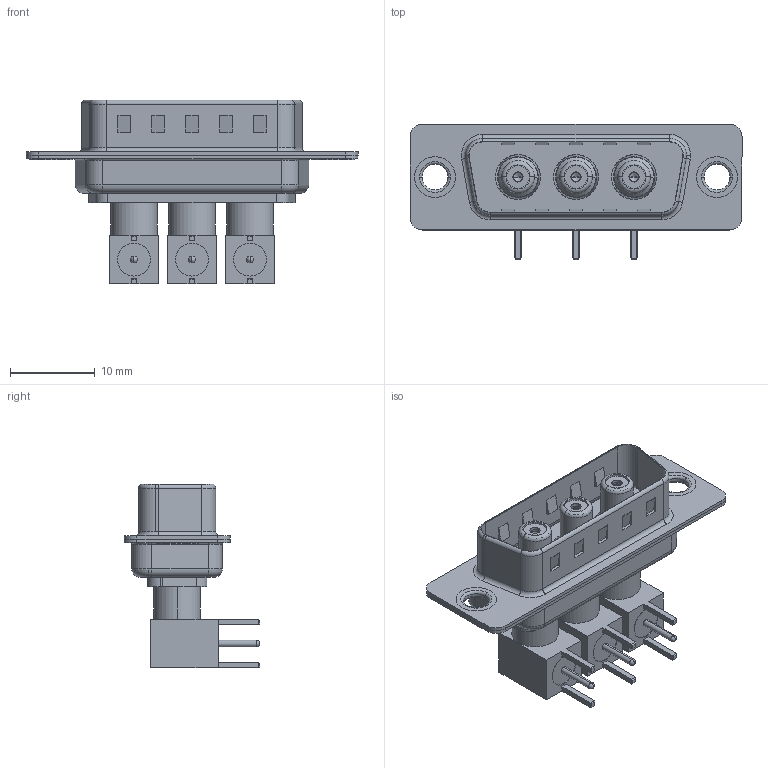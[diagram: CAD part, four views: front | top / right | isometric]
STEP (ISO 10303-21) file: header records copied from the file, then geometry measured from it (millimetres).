
FILE_DESCRIPTION (( 'STEP AP203' ), '1' );
FILE_NAME ('629-3W3-640-7T1.STEP', '2022-05-05T06:26:25', ( '' ), ( '' ), 'SwSTEP 2.0', 'SolidWorks 2020', '' );
FILE_SCHEMA (( 'CONFIG_CONTROL_DESIGN' ));
Length unit declared in the file: millimetre
Products named in the file (15): RA Back Shell; Locking Collar; Co-Ax Jack_RA PC Tail; 629-3W3-640-7T1; Co-Ax Jack Assy_RA; 629Combo Shell Rear_15 Contacts; Insulator RA Pin; Socket_RA; 629Combo Housing_3W3; 629Combo Thru Hole Rivet; Insulator Socket; Insulator Socket 2; 629Combo Shell Front_15 Contacts
Assembly tree (29 placements, depth 3):
  629-3W3-640-7T1
    629Combo Housing_3W3
    629Combo Shell Rear_15 Contacts
    629Combo Shell Front_15 Contacts
    629Combo Thru Hole Rivet  x2
    Co-Ax Jack Assy_RA
      Co-Ax Jack_RA PC Tail
      Insulator Socket
      Insulator Socket 2
      Locking Collar
      Socket_RA
      RA Back Shell
      Insulator RA Pin
    Co-Ax Jack Assy_RA
      Co-Ax Jack_RA PC Tail
      Insulator Socket
      Insulator Socket 2
      Locking Collar
      Socket_RA
      RA Back Shell
      Insulator RA Pin
    Co-Ax Jack Assy_RA
      Co-Ax Jack_RA PC Tail
      Insulator Socket
      Insulator Socket 2
      Locking Collar
      Socket_RA
      RA Back Shell
      Insulator RA Pin
Bounding box: 39.2 x 16 x 21.71 mm (x, y, z)
Volume: 2619.6 mm3; surface area: 7377.7 mm2
Topology: 26 solids, 26 shells, 770 faces, 1810 edges, 1121 vertices
Faces by surface type: cylinder 318, plane 310, torus 76, cone 57, sphere 6, bspline 3
Entity records: 15620 total; most frequent: CARTESIAN_POINT 2527, DIRECTION 2501, ORIENTED_EDGE 2184, EDGE_CURVE 1092, AXIS2_PLACEMENT_3D 952, VERTEX_POINT 685, VECTOR 597, LINE 597
